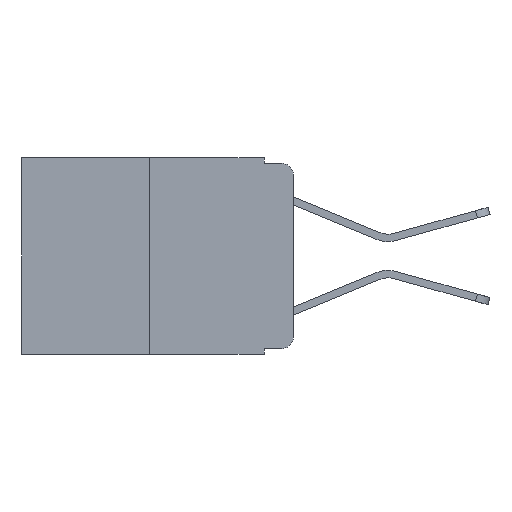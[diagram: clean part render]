
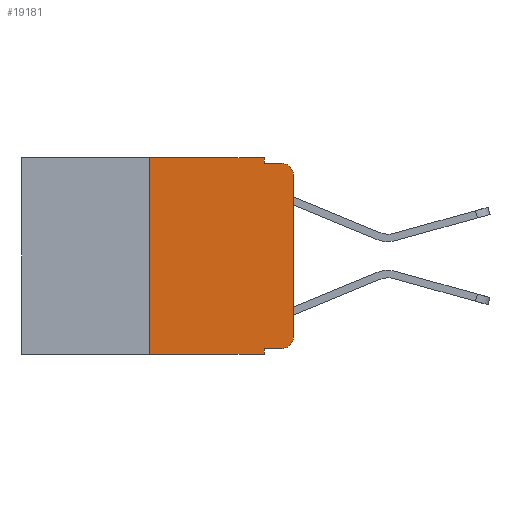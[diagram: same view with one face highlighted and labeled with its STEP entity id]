
A CAD part, left-side view. The second image highlights one B-rep face of the part: STEP entity #19181.
In plain terms, the highlighted planar face has unit normal (-1, 0, 0).
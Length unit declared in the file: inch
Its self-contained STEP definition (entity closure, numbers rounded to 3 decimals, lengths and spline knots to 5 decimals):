
#197 = LINE ( 'NONE', #6953, #5195 ) ;
#355 = VECTOR ( 'NONE', #18057, 39.37008 ) ;
#508 = VERTEX_POINT ( 'NONE', #4801 ) ;
#1146 = DIRECTION ( 'NONE',  ( 0., 0., -1. ) ) ;
#1469 = CARTESIAN_POINT ( 'NONE',  ( 0., 0.02, -0.333 ) ) ;
#2944 = VECTOR ( 'NONE', #7591, 39.37008 ) ;
#3221 = EDGE_CURVE ( 'NONE', #5859, #4271, #23788, .T. ) ;
#3280 = CARTESIAN_POINT ( 'NONE',  ( 0., 0.051, 0. ) ) ;
#3405 = CARTESIAN_POINT ( 'NONE',  ( 0., 0.473, -0.343 ) ) ;
#3443 = VERTEX_POINT ( 'NONE', #7742 ) ;
#3834 = CARTESIAN_POINT ( 'NONE',  ( 0., 0.473, 0. ) ) ;
#3916 = EDGE_LOOP ( 'NONE', ( #6974, #17485, #12804, #18113, #13435, #18713, #19331, #9475, #19970, #10102 ) ) ;
#4021 = FACE_OUTER_BOUND ( 'NONE', #3916, .T. ) ;
#4271 = VERTEX_POINT ( 'NONE', #22014 ) ;
#4442 = LINE ( 'NONE', #3280, #19723 ) ;
#4773 = VERTEX_POINT ( 'NONE', #1469 ) ;
#4801 = CARTESIAN_POINT ( 'NONE',  ( 0., 0.051, -0.333 ) ) ;
#5026 = VECTOR ( 'NONE', #19531, 39.37008 ) ;
#5087 = CARTESIAN_POINT ( 'NONE',  ( 0., 0.02, -0.313 ) ) ;
#5195 = VECTOR ( 'NONE', #22745, 39.37008 ) ;
#5438 = VERTEX_POINT ( 'NONE', #25556 ) ;
#5533 = CARTESIAN_POINT ( 'NONE',  ( 0., 0.25, 0. ) ) ;
#5859 = VERTEX_POINT ( 'NONE', #24856 ) ;
#6018 = LINE ( 'NONE', #6198, #355 ) ;
#6198 = CARTESIAN_POINT ( 'NONE',  ( 0., 0.051, -0.01 ) ) ;
#6953 = CARTESIAN_POINT ( 'NONE',  ( 0., 0.051, -0.333 ) ) ;
#6974 = ORIENTED_EDGE ( 'NONE', *, *, #25560, .T. ) ;
#7171 = DIRECTION ( 'NONE',  ( 0., 0., -1. ) ) ;
#7293 = VERTEX_POINT ( 'NONE', #19120 ) ;
#7591 = DIRECTION ( 'NONE',  ( 0., 0., 1. ) ) ;
#7676 = AXIS2_PLACEMENT_3D ( 'NONE', #3834, #7995, #21798 ) ;
#7742 = CARTESIAN_POINT ( 'NONE',  ( 0., 0.051, 0. ) ) ;
#7995 = DIRECTION ( 'NONE',  ( 1., 0., 0. ) ) ;
#8046 = VECTOR ( 'NONE', #11218, 39.37008 ) ;
#9475 = ORIENTED_EDGE ( 'NONE', *, *, #18983, .F. ) ;
#9773 = LINE ( 'NONE', #13626, #5026 ) ;
#9883 = CARTESIAN_POINT ( 'NONE',  ( 0., 0.25, 0. ) ) ;
#9972 = VECTOR ( 'NONE', #25366, 39.37008 ) ;
#10102 = ORIENTED_EDGE ( 'NONE', *, *, #15006, .T. ) ;
#10374 = VERTEX_POINT ( 'NONE', #9883 ) ;
#11218 = DIRECTION ( 'NONE',  ( 0., -1., 0. ) ) ;
#11291 = DIRECTION ( 'NONE',  ( -1., 0., 0. ) ) ;
#12107 = LINE ( 'NONE', #17053, #22005 ) ;
#12493 = AXIS2_PLACEMENT_3D ( 'NONE', #23113, #11291, #25079 ) ;
#12804 = ORIENTED_EDGE ( 'NONE', *, *, #22948, .F. ) ;
#13398 = CIRCLE ( 'NONE', #12493, 0.02 ) ;
#13435 = ORIENTED_EDGE ( 'NONE', *, *, #22781, .F. ) ;
#13626 = CARTESIAN_POINT ( 'NONE',  ( 0., 0.473, 0. ) ) ;
#13816 = PLANE ( 'NONE',  #7676 ) ;
#14329 = CARTESIAN_POINT ( 'NONE',  ( 0., 0., -0.03 ) ) ;
#15006 = EDGE_CURVE ( 'NONE', #4773, #21751, #25931, .T. ) ;
#15829 = LINE ( 'NONE', #23413, #9972 ) ;
#17053 = CARTESIAN_POINT ( 'NONE',  ( 0., 0., 0. ) ) ;
#17485 = ORIENTED_EDGE ( 'NONE', *, *, #24239, .T. ) ;
#17665 = EDGE_CURVE ( 'NONE', #508, #4773, #197, .T. ) ;
#17685 = AXIS2_PLACEMENT_3D ( 'NONE', #5087, #18988, #7171 ) ;
#18057 = DIRECTION ( 'NONE',  ( 0., -1., 0. ) ) ;
#18113 = ORIENTED_EDGE ( 'NONE', *, *, #21637, .F. ) ;
#18713 = ORIENTED_EDGE ( 'NONE', *, *, #20282, .F. ) ;
#18938 = LINE ( 'NONE', #5533, #2944 ) ;
#18983 = EDGE_CURVE ( 'NONE', #508, #4271, #4442, .T. ) ;
#18988 = DIRECTION ( 'NONE',  ( -1., 0., 0. ) ) ;
#19043 = DIRECTION ( 'NONE',  ( 0., 0., 1. ) ) ;
#19120 = CARTESIAN_POINT ( 'NONE',  ( 0., 0.051, -0.01 ) ) ;
#19181 = ADVANCED_FACE ( 'NONE', ( #4021 ), #13816, .F. ) ;
#19331 = ORIENTED_EDGE ( 'NONE', *, *, #3221, .T. ) ;
#19531 = DIRECTION ( 'NONE',  ( 0., -1., 0. ) ) ;
#19723 = VECTOR ( 'NONE', #1146, 39.37008 ) ;
#19970 = ORIENTED_EDGE ( 'NONE', *, *, #17665, .T. ) ;
#20282 = EDGE_CURVE ( 'NONE', #5859, #10374, #18938, .T. ) ;
#21637 = EDGE_CURVE ( 'NONE', #3443, #7293, #15829, .T. ) ;
#21751 = VERTEX_POINT ( 'NONE', #23752 ) ;
#21798 = DIRECTION ( 'NONE',  ( 0., 0., -1. ) ) ;
#22005 = VECTOR ( 'NONE', #19043, 39.37008 ) ;
#22014 = CARTESIAN_POINT ( 'NONE',  ( 0., 0.051, -0.343 ) ) ;
#22745 = DIRECTION ( 'NONE',  ( 0., -1., 0. ) ) ;
#22781 = EDGE_CURVE ( 'NONE', #10374, #3443, #9773, .T. ) ;
#22948 = EDGE_CURVE ( 'NONE', #7293, #5438, #6018, .T. ) ;
#23113 = CARTESIAN_POINT ( 'NONE',  ( 0., 0.02, -0.03 ) ) ;
#23413 = CARTESIAN_POINT ( 'NONE',  ( 0., 0.051, 0. ) ) ;
#23752 = CARTESIAN_POINT ( 'NONE',  ( 0., 0., -0.313 ) ) ;
#23788 = LINE ( 'NONE', #3405, #8046 ) ;
#24239 = EDGE_CURVE ( 'NONE', #25967, #5438, #13398, .T. ) ;
#24856 = CARTESIAN_POINT ( 'NONE',  ( 0., 0.25, -0.343 ) ) ;
#25079 = DIRECTION ( 'NONE',  ( 0., 0., -1. ) ) ;
#25366 = DIRECTION ( 'NONE',  ( 0., 0., -1. ) ) ;
#25556 = CARTESIAN_POINT ( 'NONE',  ( 0., 0.02, -0.01 ) ) ;
#25560 = EDGE_CURVE ( 'NONE', #21751, #25967, #12107, .T. ) ;
#25931 = CIRCLE ( 'NONE', #17685, 0.02 ) ;
#25967 = VERTEX_POINT ( 'NONE', #14329 ) ;
